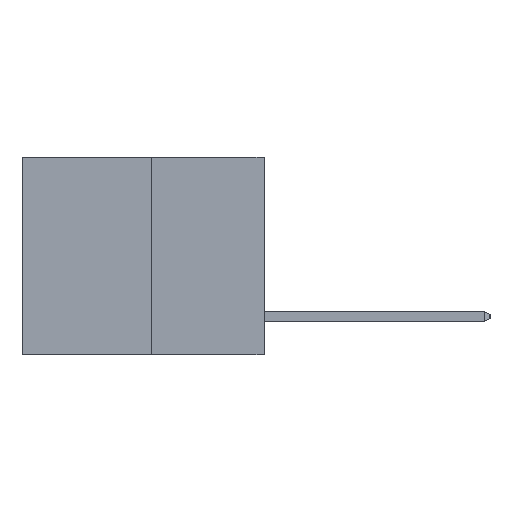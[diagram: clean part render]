
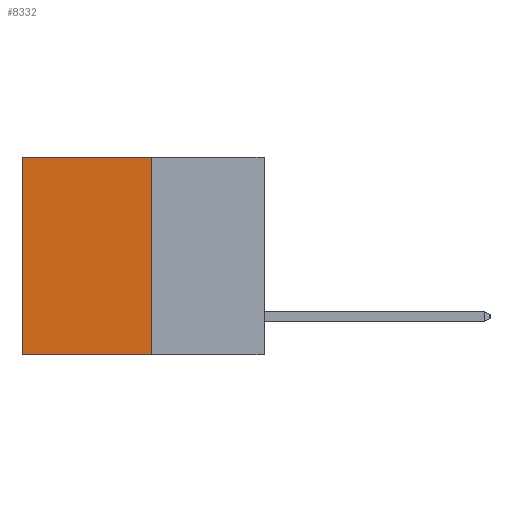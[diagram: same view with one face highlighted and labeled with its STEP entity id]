
A CAD part, left-side view. The second image highlights one B-rep face of the part: STEP entity #8332.
In plain terms, the highlighted planar face has unit normal (-1, 0, 0).
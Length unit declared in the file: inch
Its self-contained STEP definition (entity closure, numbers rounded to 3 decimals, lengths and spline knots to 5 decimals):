
#1784 = VERTEX_POINT ( 'NONE', #1936 ) ;
#1936 = CARTESIAN_POINT ( 'NONE',  ( 0.3165, 0.6, -0.49 ) ) ;
#3210 = ORIENTED_EDGE ( 'NONE', *, *, #3440, .T. ) ;
#3440 = EDGE_CURVE ( 'NONE', #15323, #1784, #23077, .T. ) ;
#4371 = CARTESIAN_POINT ( 'NONE',  ( 0.3165, 0.6, 0. ) ) ;
#4428 = DIRECTION ( 'NONE',  ( 0., 0., -1. ) ) ;
#5173 = CARTESIAN_POINT ( 'NONE',  ( 0.3165, 0.28, -0.49 ) ) ;
#5759 = DIRECTION ( 'NONE',  ( 0., 0., -1. ) ) ;
#6108 = CARTESIAN_POINT ( 'NONE',  ( 0.3165, 0.28, -0.49 ) ) ;
#6293 = EDGE_CURVE ( 'NONE', #11306, #15323, #13467, .T. ) ;
#6344 = VECTOR ( 'NONE', #11517, 39.37008 ) ;
#7815 = FACE_OUTER_BOUND ( 'NONE', #16591, .T. ) ;
#7887 = ORIENTED_EDGE ( 'NONE', *, *, #18272, .F. ) ;
#8011 = CARTESIAN_POINT ( 'NONE',  ( 0.3165, 0.6, -0.49 ) ) ;
#8332 = ADVANCED_FACE ( 'NONE', ( #7815 ), #14481, .F. ) ;
#8725 = VECTOR ( 'NONE', #15514, 39.37008 ) ;
#9653 = DIRECTION ( 'NONE',  ( 0., 0., -1. ) ) ;
#11087 = LINE ( 'NONE', #16719, #6344 ) ;
#11306 = VERTEX_POINT ( 'NONE', #14996 ) ;
#11517 = DIRECTION ( 'NONE',  ( 0., 1., 0. ) ) ;
#12135 = ORIENTED_EDGE ( 'NONE', *, *, #16423, .F. ) ;
#12649 = LINE ( 'NONE', #6108, #16853 ) ;
#13467 = LINE ( 'NONE', #22761, #8725 ) ;
#13985 = ORIENTED_EDGE ( 'NONE', *, *, #6293, .T. ) ;
#14481 = PLANE ( 'NONE',  #20710 ) ;
#14996 = CARTESIAN_POINT ( 'NONE',  ( 0.3165, 0.28, 0. ) ) ;
#15323 = VERTEX_POINT ( 'NONE', #4371 ) ;
#15514 = DIRECTION ( 'NONE',  ( 0., 1., 0. ) ) ;
#16185 = VERTEX_POINT ( 'NONE', #5173 ) ;
#16423 = EDGE_CURVE ( 'NONE', #11306, #16185, #12649, .T. ) ;
#16591 = EDGE_LOOP ( 'NONE', ( #3210, #7887, #12135, #13985 ) ) ;
#16671 = CARTESIAN_POINT ( 'NONE',  ( 0.3165, 0.28, -0.49 ) ) ;
#16719 = CARTESIAN_POINT ( 'NONE',  ( 0.3165, 0.28, -0.49 ) ) ;
#16853 = VECTOR ( 'NONE', #9653, 39.37008 ) ;
#18272 = EDGE_CURVE ( 'NONE', #16185, #1784, #11087, .T. ) ;
#18319 = VECTOR ( 'NONE', #4428, 39.37008 ) ;
#18496 = DIRECTION ( 'NONE',  ( 1., 0., 0. ) ) ;
#20710 = AXIS2_PLACEMENT_3D ( 'NONE', #16671, #18496, #5759 ) ;
#22761 = CARTESIAN_POINT ( 'NONE',  ( 0.3165, 0.28, 0. ) ) ;
#23077 = LINE ( 'NONE', #8011, #18319 ) ;
